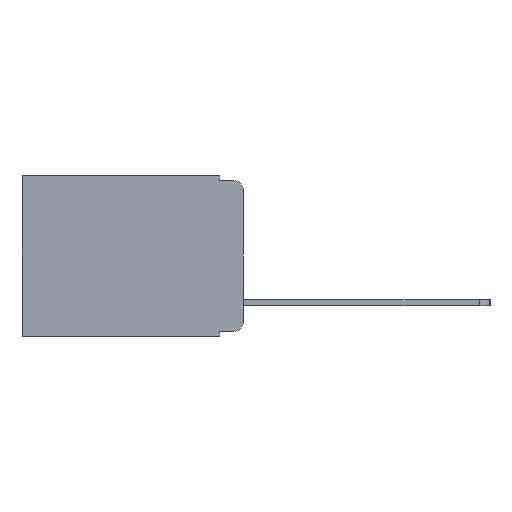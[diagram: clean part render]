
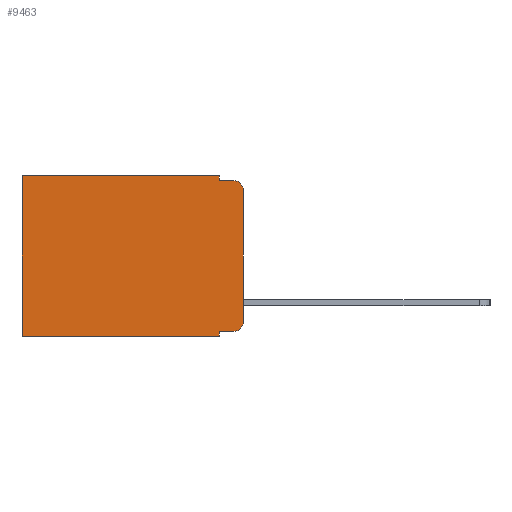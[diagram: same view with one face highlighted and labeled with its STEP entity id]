
A CAD part, left-side view. The second image highlights one B-rep face of the part: STEP entity #9463.
In plain terms, the highlighted planar face has unit normal (-1, 0, 0).
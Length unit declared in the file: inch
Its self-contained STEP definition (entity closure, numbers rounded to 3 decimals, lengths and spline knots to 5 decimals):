
#14 = ORIENTED_EDGE ( 'NONE', *, *, #19581, .F. ) ;
#71 = CARTESIAN_POINT ( 'NONE',  ( 0.298, 0.051, -0.01 ) ) ;
#127 = CARTESIAN_POINT ( 'NONE',  ( 0.298, 0., 0. ) ) ;
#313 = CIRCLE ( 'NONE', #8249, 0.02 ) ;
#467 = AXIS2_PLACEMENT_3D ( 'NONE', #5134, #2031, #12865 ) ;
#799 = LINE ( 'NONE', #17558, #5336 ) ;
#828 = EDGE_CURVE ( 'NONE', #10388, #19029, #12940, .T. ) ;
#900 = EDGE_LOOP ( 'NONE', ( #15306, #7758, #8300, #17191, #3534, #6407, #8045, #14, #4603, #10168 ) ) ;
#1402 = CARTESIAN_POINT ( 'NONE',  ( 0.298, 0.051, -0.333 ) ) ;
#1991 = EDGE_CURVE ( 'NONE', #20731, #13814, #4080, .T. ) ;
#2031 = DIRECTION ( 'NONE',  ( -1., 0., 0. ) ) ;
#2184 = CARTESIAN_POINT ( 'NONE',  ( 0.298, 0.473, 0. ) ) ;
#2429 = CARTESIAN_POINT ( 'NONE',  ( 0.298, 0., -0.343 ) ) ;
#2710 = VERTEX_POINT ( 'NONE', #12858 ) ;
#2894 = CARTESIAN_POINT ( 'NONE',  ( 0.298, 0.02, -0.01 ) ) ;
#3029 = VERTEX_POINT ( 'NONE', #1402 ) ;
#3030 = VERTEX_POINT ( 'NONE', #2894 ) ;
#3050 = DIRECTION ( 'NONE',  ( 0., 0., -1. ) ) ;
#3132 = EDGE_CURVE ( 'NONE', #13814, #3030, #3196, .T. ) ;
#3196 = LINE ( 'NONE', #71, #15728 ) ;
#3227 = DIRECTION ( 'NONE',  ( 0., -1., 0. ) ) ;
#3534 = ORIENTED_EDGE ( 'NONE', *, *, #5449, .T. ) ;
#3783 = LINE ( 'NONE', #5537, #4312 ) ;
#4080 = LINE ( 'NONE', #14957, #13427 ) ;
#4172 = DIRECTION ( 'NONE',  ( 0., 1., 0. ) ) ;
#4289 = EDGE_CURVE ( 'NONE', #7761, #3030, #16144, .T. ) ;
#4312 = VECTOR ( 'NONE', #7230, 39.37008 ) ;
#4603 = ORIENTED_EDGE ( 'NONE', *, *, #18603, .T. ) ;
#4619 = CARTESIAN_POINT ( 'NONE',  ( 0.298, 0.051, 0. ) ) ;
#4885 = VECTOR ( 'NONE', #3227, 39.37008 ) ;
#5134 = CARTESIAN_POINT ( 'NONE',  ( 0.298, 0.02, -0.03 ) ) ;
#5336 = VECTOR ( 'NONE', #3050, 39.37008 ) ;
#5449 = EDGE_CURVE ( 'NONE', #20731, #10388, #10229, .T. ) ;
#5537 = CARTESIAN_POINT ( 'NONE',  ( 0.298, 0.051, 0. ) ) ;
#6201 = CARTESIAN_POINT ( 'NONE',  ( 0.298, 0., 0. ) ) ;
#6407 = ORIENTED_EDGE ( 'NONE', *, *, #828, .T. ) ;
#6740 = CARTESIAN_POINT ( 'NONE',  ( 0.298, 0., -0.03 ) ) ;
#7230 = DIRECTION ( 'NONE',  ( 0., 0., -1. ) ) ;
#7673 = EDGE_CURVE ( 'NONE', #7761, #2710, #799, .T. ) ;
#7758 = ORIENTED_EDGE ( 'NONE', *, *, #4289, .T. ) ;
#7761 = VERTEX_POINT ( 'NONE', #6740 ) ;
#7845 = VERTEX_POINT ( 'NONE', #8678 ) ;
#7944 = DIRECTION ( 'NONE',  ( 0., 0., -1. ) ) ;
#8045 = ORIENTED_EDGE ( 'NONE', *, *, #10918, .F. ) ;
#8249 = AXIS2_PLACEMENT_3D ( 'NONE', #10146, #20776, #11785 ) ;
#8300 = ORIENTED_EDGE ( 'NONE', *, *, #3132, .F. ) ;
#8533 = DIRECTION ( 'NONE',  ( 0., -1., 0. ) ) ;
#8556 = VERTEX_POINT ( 'NONE', #13779 ) ;
#8678 = CARTESIAN_POINT ( 'NONE',  ( 0.298, 0.051, -0.343 ) ) ;
#9463 = ADVANCED_FACE ( 'NONE', ( #19806 ), #12821, .F. ) ;
#10080 = CARTESIAN_POINT ( 'NONE',  ( 0.298, 0.473, 0. ) ) ;
#10146 = CARTESIAN_POINT ( 'NONE',  ( 0.298, 0.02, -0.313 ) ) ;
#10168 = ORIENTED_EDGE ( 'NONE', *, *, #16608, .T. ) ;
#10229 = LINE ( 'NONE', #127, #17965 ) ;
#10388 = VERTEX_POINT ( 'NONE', #2184 ) ;
#10687 = VECTOR ( 'NONE', #4172, 39.37008 ) ;
#10735 = DIRECTION ( 'NONE',  ( 0., 0., -1. ) ) ;
#10918 = EDGE_CURVE ( 'NONE', #7845, #19029, #14863, .T. ) ;
#11785 = DIRECTION ( 'NONE',  ( 0., 0., -1. ) ) ;
#12423 = VECTOR ( 'NONE', #18739, 39.37008 ) ;
#12821 = PLANE ( 'NONE',  #19009 ) ;
#12858 = CARTESIAN_POINT ( 'NONE',  ( 0.298, 0., -0.313 ) ) ;
#12865 = DIRECTION ( 'NONE',  ( 0., 0., -1. ) ) ;
#12940 = LINE ( 'NONE', #10080, #12423 ) ;
#13427 = VECTOR ( 'NONE', #10735, 39.37008 ) ;
#13696 = LINE ( 'NONE', #14769, #4885 ) ;
#13779 = CARTESIAN_POINT ( 'NONE',  ( 0.298, 0.02, -0.333 ) ) ;
#13814 = VERTEX_POINT ( 'NONE', #14835 ) ;
#14357 = CARTESIAN_POINT ( 'NONE',  ( 0.298, 0.473, -0.343 ) ) ;
#14769 = CARTESIAN_POINT ( 'NONE',  ( 0.298, 0.051, -0.333 ) ) ;
#14835 = CARTESIAN_POINT ( 'NONE',  ( 0.298, 0.051, -0.01 ) ) ;
#14863 = LINE ( 'NONE', #2429, #10687 ) ;
#14957 = CARTESIAN_POINT ( 'NONE',  ( 0.298, 0.051, 0. ) ) ;
#15306 = ORIENTED_EDGE ( 'NONE', *, *, #7673, .F. ) ;
#15728 = VECTOR ( 'NONE', #8533, 39.37008 ) ;
#16144 = CIRCLE ( 'NONE', #467, 0.02 ) ;
#16608 = EDGE_CURVE ( 'NONE', #8556, #2710, #313, .T. ) ;
#17004 = DIRECTION ( 'NONE',  ( 0., 1., 0. ) ) ;
#17191 = ORIENTED_EDGE ( 'NONE', *, *, #1991, .F. ) ;
#17412 = DIRECTION ( 'NONE',  ( 1., 0., 0. ) ) ;
#17558 = CARTESIAN_POINT ( 'NONE',  ( 0.298, 0., 0. ) ) ;
#17965 = VECTOR ( 'NONE', #17004, 39.37008 ) ;
#18603 = EDGE_CURVE ( 'NONE', #3029, #8556, #13696, .T. ) ;
#18739 = DIRECTION ( 'NONE',  ( 0., 0., -1. ) ) ;
#19009 = AXIS2_PLACEMENT_3D ( 'NONE', #6201, #17412, #7944 ) ;
#19029 = VERTEX_POINT ( 'NONE', #14357 ) ;
#19581 = EDGE_CURVE ( 'NONE', #3029, #7845, #3783, .T. ) ;
#19806 = FACE_OUTER_BOUND ( 'NONE', #900, .T. ) ;
#20731 = VERTEX_POINT ( 'NONE', #4619 ) ;
#20776 = DIRECTION ( 'NONE',  ( -1., 0., 0. ) ) ;
